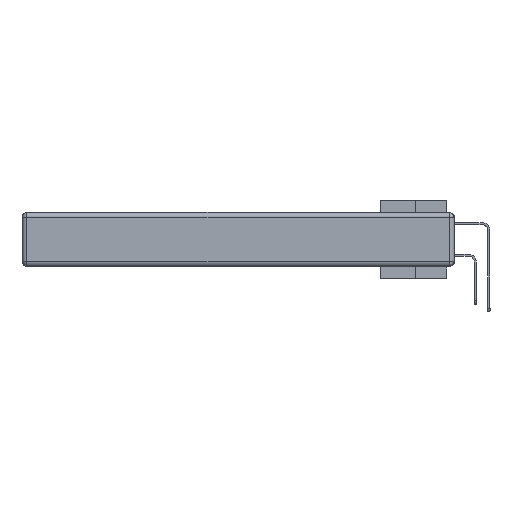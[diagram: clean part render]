
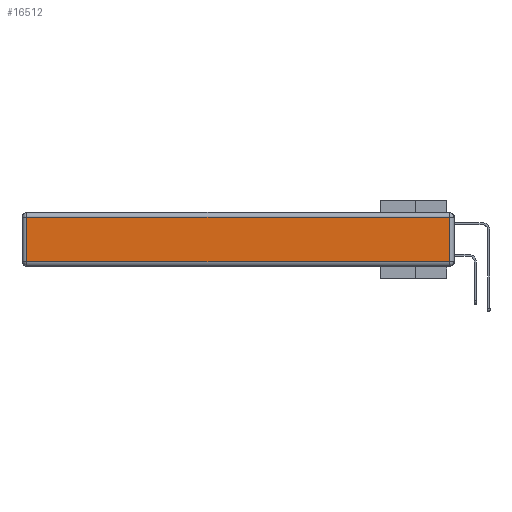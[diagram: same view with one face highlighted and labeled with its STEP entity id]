
A CAD part, left-side view. The second image highlights one B-rep face of the part: STEP entity #16512.
In plain terms, the highlighted planar face has unit normal (-1, 0, 0).
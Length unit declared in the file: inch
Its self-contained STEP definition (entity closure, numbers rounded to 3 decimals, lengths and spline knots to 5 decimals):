
#307 = DIRECTION ( 'NONE',  ( 0., 0., 1. ) ) ;
#472 = CARTESIAN_POINT ( 'NONE',  ( 0., 0.03, -0.343 ) ) ;
#1486 = EDGE_CURVE ( 'NONE', #9783, #6267, #9995, .T. ) ;
#2552 = CARTESIAN_POINT ( 'NONE',  ( 0., 2.72, -0.313 ) ) ;
#3897 = LINE ( 'NONE', #11453, #7512 ) ;
#3917 = FACE_OUTER_BOUND ( 'NONE', #19105, .T. ) ;
#5501 = VECTOR ( 'NONE', #307, 39.37008 ) ;
#6267 = VERTEX_POINT ( 'NONE', #24155 ) ;
#6274 = CARTESIAN_POINT ( 'NONE',  ( 0., 0.03, -0.313 ) ) ;
#7512 = VECTOR ( 'NONE', #31438, 39.37008 ) ;
#7777 = VERTEX_POINT ( 'NONE', #2552 ) ;
#8353 = PLANE ( 'NONE',  #28083 ) ;
#9145 = ORIENTED_EDGE ( 'NONE', *, *, #19733, .T. ) ;
#9783 = VERTEX_POINT ( 'NONE', #6274 ) ;
#9995 = LINE ( 'NONE', #472, #5501 ) ;
#10661 = VECTOR ( 'NONE', #17729, 39.37008 ) ;
#10984 = DIRECTION ( 'NONE',  ( -1., 0., 0. ) ) ;
#11453 = CARTESIAN_POINT ( 'NONE',  ( 0., 2.72, -0.343 ) ) ;
#11652 = EDGE_CURVE ( 'NONE', #6267, #25518, #29539, .T. ) ;
#12889 = ORIENTED_EDGE ( 'NONE', *, *, #11652, .T. ) ;
#13621 = CARTESIAN_POINT ( 'NONE',  ( 0., 0., -0.343 ) ) ;
#13775 = EDGE_CURVE ( 'NONE', #25518, #7777, #3897, .T. ) ;
#13793 = CARTESIAN_POINT ( 'NONE',  ( 0., 2.72, -0.03 ) ) ;
#15717 = ORIENTED_EDGE ( 'NONE', *, *, #13775, .T. ) ;
#16512 = ADVANCED_FACE ( 'NONE', ( #3917 ), #8353, .T. ) ;
#17729 = DIRECTION ( 'NONE',  ( 0., 1., 0. ) ) ;
#19105 = EDGE_LOOP ( 'NONE', ( #9145, #25386, #12889, #15717 ) ) ;
#19552 = CARTESIAN_POINT ( 'NONE',  ( 0., 2.75, -0.03 ) ) ;
#19594 = CARTESIAN_POINT ( 'NONE',  ( 0., 0., -0.313 ) ) ;
#19733 = EDGE_CURVE ( 'NONE', #7777, #9783, #26626, .T. ) ;
#23910 = DIRECTION ( 'NONE',  ( 0., 0., 1. ) ) ;
#24155 = CARTESIAN_POINT ( 'NONE',  ( 0., 0.03, -0.03 ) ) ;
#25386 = ORIENTED_EDGE ( 'NONE', *, *, #1486, .T. ) ;
#25518 = VERTEX_POINT ( 'NONE', #13793 ) ;
#26626 = LINE ( 'NONE', #19594, #27114 ) ;
#27114 = VECTOR ( 'NONE', #27117, 39.37008 ) ;
#27117 = DIRECTION ( 'NONE',  ( 0., -1., 0. ) ) ;
#28083 = AXIS2_PLACEMENT_3D ( 'NONE', #13621, #10984, #23910 ) ;
#29539 = LINE ( 'NONE', #19552, #10661 ) ;
#31438 = DIRECTION ( 'NONE',  ( 0., 0., -1. ) ) ;
